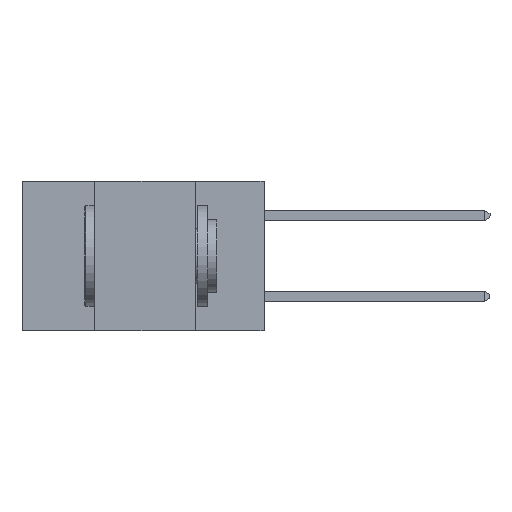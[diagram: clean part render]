
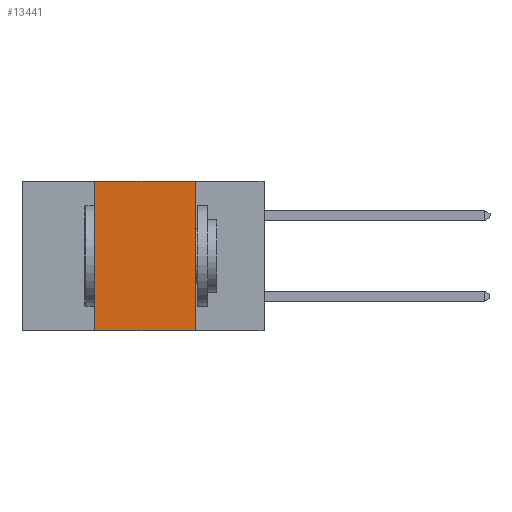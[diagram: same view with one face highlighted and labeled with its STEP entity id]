
A CAD part, left-side view. The second image highlights one B-rep face of the part: STEP entity #13441.
In plain terms, the highlighted planar face has unit normal (-1, 0, 0).
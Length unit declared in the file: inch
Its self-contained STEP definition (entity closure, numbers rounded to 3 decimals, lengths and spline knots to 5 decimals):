
#36 = VERTEX_POINT ( 'NONE', #3729 ) ;
#132 = CARTESIAN_POINT ( 'NONE',  ( 0., 0.17, 0. ) ) ;
#418 = VERTEX_POINT ( 'NONE', #132 ) ;
#935 = EDGE_CURVE ( 'NONE', #36, #418, #3810, .T. ) ;
#1207 = EDGE_LOOP ( 'NONE', ( #10049, #14060, #3587, #14922 ) ) ;
#1272 = EDGE_CURVE ( 'NONE', #4215, #16431, #9015, .T. ) ;
#1871 = CARTESIAN_POINT ( 'NONE',  ( 0., 0.6, 0. ) ) ;
#2181 = VECTOR ( 'NONE', #10112, 39.37008 ) ;
#2439 = VECTOR ( 'NONE', #2750, 39.37008 ) ;
#2530 = CARTESIAN_POINT ( 'NONE',  ( 0., 0.6, 0. ) ) ;
#2750 = DIRECTION ( 'NONE',  ( 0., 0., -1. ) ) ;
#3232 = CARTESIAN_POINT ( 'NONE',  ( 0., 0.42, 0. ) ) ;
#3587 = ORIENTED_EDGE ( 'NONE', *, *, #15579, .F. ) ;
#3729 = CARTESIAN_POINT ( 'NONE',  ( 0., 0.42, 0. ) ) ;
#3810 = LINE ( 'NONE', #1871, #16997 ) ;
#4215 = VERTEX_POINT ( 'NONE', #13075 ) ;
#5425 = DIRECTION ( 'NONE',  ( 1., 0., 0. ) ) ;
#6030 = LINE ( 'NONE', #3232, #2181 ) ;
#6438 = CARTESIAN_POINT ( 'NONE',  ( 0., 0.17, -0.37 ) ) ;
#6704 = FACE_OUTER_BOUND ( 'NONE', #1207, .T. ) ;
#8734 = CARTESIAN_POINT ( 'NONE',  ( 0., 0.6, -0.37 ) ) ;
#9015 = LINE ( 'NONE', #8734, #15368 ) ;
#10049 = ORIENTED_EDGE ( 'NONE', *, *, #15367, .F. ) ;
#10112 = DIRECTION ( 'NONE',  ( 0., 0., 1. ) ) ;
#11039 = CARTESIAN_POINT ( 'NONE',  ( 0., 0.17, 0. ) ) ;
#12945 = AXIS2_PLACEMENT_3D ( 'NONE', #2530, #5425, #14939 ) ;
#13075 = CARTESIAN_POINT ( 'NONE',  ( 0., 0.42, -0.37 ) ) ;
#13441 = ADVANCED_FACE ( 'NONE', ( #6704 ), #13579, .F. ) ;
#13579 = PLANE ( 'NONE',  #12945 ) ;
#14060 = ORIENTED_EDGE ( 'NONE', *, *, #935, .F. ) ;
#14922 = ORIENTED_EDGE ( 'NONE', *, *, #1272, .T. ) ;
#14939 = DIRECTION ( 'NONE',  ( 0., 0., -1. ) ) ;
#15367 = EDGE_CURVE ( 'NONE', #418, #16431, #16619, .T. ) ;
#15368 = VECTOR ( 'NONE', #15548, 39.37008 ) ;
#15548 = DIRECTION ( 'NONE',  ( 0., -1., 0. ) ) ;
#15579 = EDGE_CURVE ( 'NONE', #4215, #36, #6030, .T. ) ;
#16431 = VERTEX_POINT ( 'NONE', #6438 ) ;
#16619 = LINE ( 'NONE', #11039, #2439 ) ;
#16997 = VECTOR ( 'NONE', #17275, 39.37008 ) ;
#17275 = DIRECTION ( 'NONE',  ( 0., -1., 0. ) ) ;
